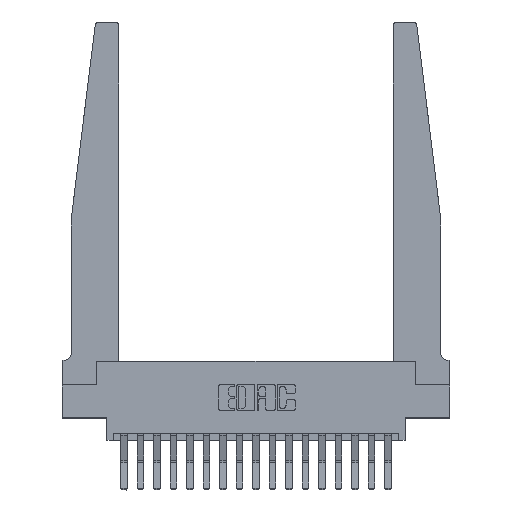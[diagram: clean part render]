
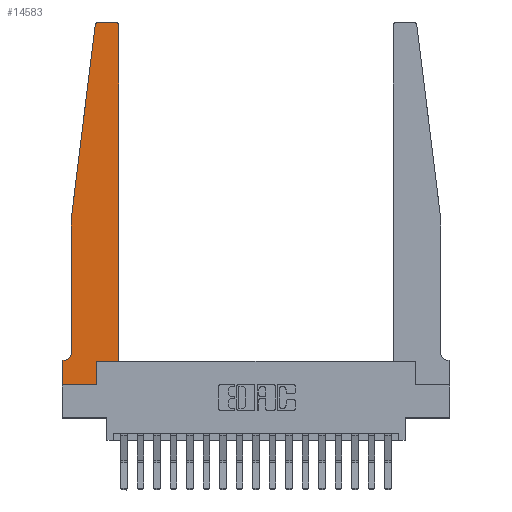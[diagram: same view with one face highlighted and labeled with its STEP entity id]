
A CAD part, top view. The second image highlights one B-rep face of the part: STEP entity #14583.
In plain terms, the highlighted planar face has unit normal (0, 0, 1).
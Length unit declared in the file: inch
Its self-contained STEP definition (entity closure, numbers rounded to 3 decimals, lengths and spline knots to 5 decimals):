
#633 = DIRECTION ( 'NONE',  ( 0., -1., 0. ) ) ;
#762 = VERTEX_POINT ( 'NONE', #5158 ) ;
#1128 = LINE ( 'NONE', #16975, #4186 ) ;
#1350 = AXIS2_PLACEMENT_3D ( 'NONE', #15642, #6566, #17139 ) ;
#1425 = EDGE_CURVE ( 'NONE', #15108, #3184, #16040, .T. ) ;
#1466 = ORIENTED_EDGE ( 'NONE', *, *, #10825, .T. ) ;
#1470 = VECTOR ( 'NONE', #18996, 39.37008 ) ;
#1581 = VERTEX_POINT ( 'NONE', #8471 ) ;
#1896 = ORIENTED_EDGE ( 'NONE', *, *, #9435, .T. ) ;
#2341 = DIRECTION ( 'NONE',  ( 0., 1., 0. ) ) ;
#2554 = CIRCLE ( 'NONE', #6445, 0.03 ) ;
#2717 = EDGE_CURVE ( 'NONE', #13168, #8345, #15768, .T. ) ;
#2801 = CARTESIAN_POINT ( 'NONE',  ( 0.425, 0.18, 0.37 ) ) ;
#2937 = DIRECTION ( 'NONE',  ( 1., 0., 0. ) ) ;
#3077 = EDGE_CURVE ( 'NONE', #3184, #3822, #18549, .T. ) ;
#3103 = VECTOR ( 'NONE', #19268, 39.37008 ) ;
#3158 = VERTEX_POINT ( 'NONE', #4986 ) ;
#3184 = VERTEX_POINT ( 'NONE', #3559 ) ;
#3202 = VECTOR ( 'NONE', #633, 39.37008 ) ;
#3265 = CARTESIAN_POINT ( 'NONE',  ( 0.425, 2.72, 0.37 ) ) ;
#3559 = CARTESIAN_POINT ( 'NONE',  ( 0., 0.1875, 0.37 ) ) ;
#3822 = VERTEX_POINT ( 'NONE', #17208 ) ;
#3904 = LINE ( 'NONE', #12798, #15455 ) ;
#3930 = ORIENTED_EDGE ( 'NONE', *, *, #1425, .T. ) ;
#4186 = VECTOR ( 'NONE', #9416, 39.37008 ) ;
#4445 = EDGE_CURVE ( 'NONE', #5987, #11431, #3904, .T. ) ;
#4654 = VECTOR ( 'NONE', #2937, 39.37008 ) ;
#4986 = CARTESIAN_POINT ( 'NONE',  ( 0.27653, 2.75, 0.37 ) ) ;
#5140 = DIRECTION ( 'NONE',  ( -1., 0., 0. ) ) ;
#5158 = CARTESIAN_POINT ( 'NONE',  ( 0.395, 2.75, 0.37 ) ) ;
#5912 = LINE ( 'NONE', #6952, #1470 ) ;
#5987 = VERTEX_POINT ( 'NONE', #2801 ) ;
#6092 = DIRECTION ( 'NONE',  ( 0., -1., 0. ) ) ;
#6445 = AXIS2_PLACEMENT_3D ( 'NONE', #8598, #19121, #10093 ) ;
#6521 = CARTESIAN_POINT ( 'NONE',  ( 0., 0.1875, 0.37 ) ) ;
#6566 = DIRECTION ( 'NONE',  ( 0., 0., -1. ) ) ;
#6630 = VERTEX_POINT ( 'NONE', #10270 ) ;
#6864 = ORIENTED_EDGE ( 'NONE', *, *, #14531, .T. ) ;
#6952 = CARTESIAN_POINT ( 'NONE',  ( 0.25, 2.75, 0.37 ) ) ;
#7046 = LINE ( 'NONE', #17793, #3103 ) ;
#7200 = FACE_OUTER_BOUND ( 'NONE', #11677, .T. ) ;
#7312 = EDGE_CURVE ( 'NONE', #3822, #6630, #7046, .T. ) ;
#8035 = DIRECTION ( 'NONE',  ( 1., 0., 0. ) ) ;
#8345 = VERTEX_POINT ( 'NONE', #9475 ) ;
#8471 = CARTESIAN_POINT ( 'NONE',  ( 0.065, 0.2375, 0.37 ) ) ;
#8505 = CARTESIAN_POINT ( 'NONE',  ( 0.065, 1.25, 0.37 ) ) ;
#8598 = CARTESIAN_POINT ( 'NONE',  ( 0.395, 2.72, 0.37 ) ) ;
#8626 = LINE ( 'NONE', #13217, #4654 ) ;
#8728 = DIRECTION ( 'NONE',  ( 0., 0., 1. ) ) ;
#9313 = ORIENTED_EDGE ( 'NONE', *, *, #3077, .T. ) ;
#9393 = CARTESIAN_POINT ( 'NONE',  ( 0.015, 0.1875, 0.37 ) ) ;
#9416 = DIRECTION ( 'NONE',  ( 0., 1., 0. ) ) ;
#9435 = EDGE_CURVE ( 'NONE', #17983, #5987, #8626, .T. ) ;
#9475 = CARTESIAN_POINT ( 'NONE',  ( 0.065, 1.25, 0.37 ) ) ;
#9517 = ORIENTED_EDGE ( 'NONE', *, *, #4445, .T. ) ;
#9649 = CARTESIAN_POINT ( 'NONE',  ( 0.065, 1.25, 0.37 ) ) ;
#9810 = EDGE_CURVE ( 'NONE', #11431, #762, #2554, .T. ) ;
#10093 = DIRECTION ( 'NONE',  ( 1., 0., 0. ) ) ;
#10270 = CARTESIAN_POINT ( 'NONE',  ( 0.2605, 0., 0.37 ) ) ;
#10449 = CIRCLE ( 'NONE', #1350, 0.05 ) ;
#10523 = VECTOR ( 'NONE', #6092, 39.37008 ) ;
#10675 = LINE ( 'NONE', #9649, #3202 ) ;
#10825 = EDGE_CURVE ( 'NONE', #1581, #15108, #10449, .T. ) ;
#11013 = PLANE ( 'NONE',  #12299 ) ;
#11161 = ORIENTED_EDGE ( 'NONE', *, *, #2717, .T. ) ;
#11431 = VERTEX_POINT ( 'NONE', #3265 ) ;
#11554 = CIRCLE ( 'NONE', #12273, 0.03 ) ;
#11677 = EDGE_LOOP ( 'NONE', ( #12487, #15889, #11161, #12561, #1466, #3930, #9313, #18684, #6864, #1896, #9517, #15389 ) ) ;
#11726 = VECTOR ( 'NONE', #16123, 39.37008 ) ;
#11744 = EDGE_CURVE ( 'NONE', #762, #3158, #5912, .T. ) ;
#11848 = EDGE_CURVE ( 'NONE', #3158, #13168, #11554, .T. ) ;
#12273 = AXIS2_PLACEMENT_3D ( 'NONE', #17781, #8728, #19256 ) ;
#12299 = AXIS2_PLACEMENT_3D ( 'NONE', #6521, #17097, #8035 ) ;
#12459 = VECTOR ( 'NONE', #5140, 39.37008 ) ;
#12487 = ORIENTED_EDGE ( 'NONE', *, *, #11744, .T. ) ;
#12561 = ORIENTED_EDGE ( 'NONE', *, *, #16801, .T. ) ;
#12798 = CARTESIAN_POINT ( 'NONE',  ( 0.425, 0.18, 0.37 ) ) ;
#13168 = VERTEX_POINT ( 'NONE', #16176 ) ;
#13217 = CARTESIAN_POINT ( 'NONE',  ( 0.425, 0.18, 0.37 ) ) ;
#14143 = CARTESIAN_POINT ( 'NONE',  ( 0.065, 0.1875, 0.37 ) ) ;
#14531 = EDGE_CURVE ( 'NONE', #6630, #17983, #1128, .T. ) ;
#14583 = ADVANCED_FACE ( 'NONE', ( #7200 ), #11013, .T. ) ;
#15108 = VERTEX_POINT ( 'NONE', #9393 ) ;
#15389 = ORIENTED_EDGE ( 'NONE', *, *, #9810, .T. ) ;
#15455 = VECTOR ( 'NONE', #2341, 39.37008 ) ;
#15642 = CARTESIAN_POINT ( 'NONE',  ( 0.015, 0.2375, 0.37 ) ) ;
#15768 = LINE ( 'NONE', #8505, #11726 ) ;
#15889 = ORIENTED_EDGE ( 'NONE', *, *, #11848, .T. ) ;
#16040 = LINE ( 'NONE', #14143, #12459 ) ;
#16123 = DIRECTION ( 'NONE',  ( -0.122, -0.992, 0. ) ) ;
#16176 = CARTESIAN_POINT ( 'NONE',  ( 0.24675, 2.72367, 0.37 ) ) ;
#16183 = CARTESIAN_POINT ( 'NONE',  ( 0.2605, 0.18, 0.37 ) ) ;
#16649 = CARTESIAN_POINT ( 'NONE',  ( 0., 0., 0.37 ) ) ;
#16801 = EDGE_CURVE ( 'NONE', #8345, #1581, #10675, .T. ) ;
#16975 = CARTESIAN_POINT ( 'NONE',  ( 0.2605, 0.18, 0.37 ) ) ;
#17097 = DIRECTION ( 'NONE',  ( 0., 0., 1. ) ) ;
#17139 = DIRECTION ( 'NONE',  ( -1., 0., 0. ) ) ;
#17208 = CARTESIAN_POINT ( 'NONE',  ( 0., 0., 0.37 ) ) ;
#17781 = CARTESIAN_POINT ( 'NONE',  ( 0.27653, 2.72, 0.37 ) ) ;
#17793 = CARTESIAN_POINT ( 'NONE',  ( 0., 0., 0.37 ) ) ;
#17983 = VERTEX_POINT ( 'NONE', #16183 ) ;
#18549 = LINE ( 'NONE', #16649, #10523 ) ;
#18684 = ORIENTED_EDGE ( 'NONE', *, *, #7312, .T. ) ;
#18996 = DIRECTION ( 'NONE',  ( -1., 0., 0. ) ) ;
#19121 = DIRECTION ( 'NONE',  ( 0., 0., 1. ) ) ;
#19256 = DIRECTION ( 'NONE',  ( 1., 0., 0. ) ) ;
#19268 = DIRECTION ( 'NONE',  ( 1., 0., 0. ) ) ;
